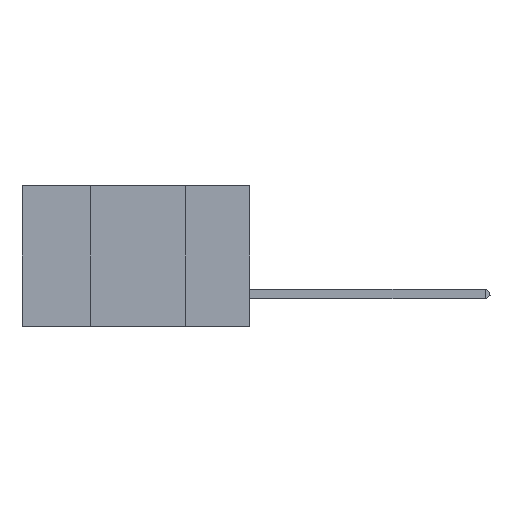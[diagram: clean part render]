
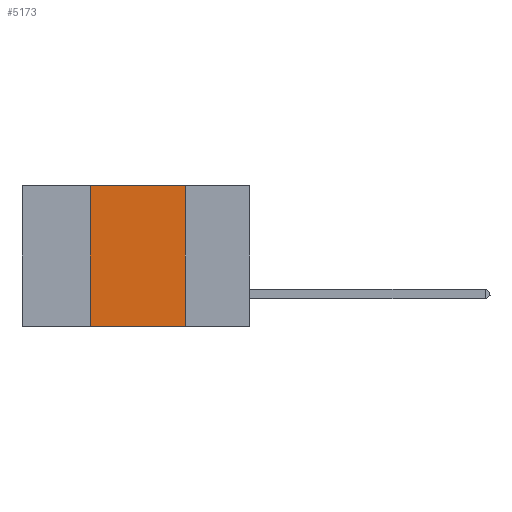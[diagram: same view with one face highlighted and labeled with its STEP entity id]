
A CAD part, left-side view. The second image highlights one B-rep face of the part: STEP entity #5173.
In plain terms, the highlighted planar face has unit normal (-1, 0, 0).
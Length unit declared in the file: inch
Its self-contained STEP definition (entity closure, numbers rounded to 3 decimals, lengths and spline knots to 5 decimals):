
#3717 = CARTESIAN_POINT ( 'NONE',  ( 0., 0.17, -0.37 ) ) ;
#4287 = ORIENTED_EDGE ( 'NONE', *, *, #43970, .F. ) ;
#4582 = PLANE ( 'NONE',  #5928 ) ;
#4859 = CARTESIAN_POINT ( 'NONE',  ( 0., 0.17, 0. ) ) ;
#5173 = ADVANCED_FACE ( 'NONE', ( #27653 ), #4582, .F. ) ;
#5928 = AXIS2_PLACEMENT_3D ( 'NONE', #19264, #23819, #9430 ) ;
#8566 = CARTESIAN_POINT ( 'NONE',  ( 0., 0.17, 0. ) ) ;
#9430 = DIRECTION ( 'NONE',  ( 0., 0., -1. ) ) ;
#11732 = VECTOR ( 'NONE', #38789, 39.37008 ) ;
#11736 = VECTOR ( 'NONE', #12236, 39.37008 ) ;
#12236 = DIRECTION ( 'NONE',  ( 0., -1., 0. ) ) ;
#12929 = VERTEX_POINT ( 'NONE', #45999 ) ;
#15854 = CARTESIAN_POINT ( 'NONE',  ( 0., 0.6, -0.37 ) ) ;
#19030 = VERTEX_POINT ( 'NONE', #3717 ) ;
#19264 = CARTESIAN_POINT ( 'NONE',  ( 0., 0.6, 0. ) ) ;
#20311 = EDGE_CURVE ( 'NONE', #21935, #45331, #34620, .T. ) ;
#21935 = VERTEX_POINT ( 'NONE', #44883 ) ;
#22115 = EDGE_CURVE ( 'NONE', #45331, #19030, #37363, .T. ) ;
#22333 = ORIENTED_EDGE ( 'NONE', *, *, #20311, .F. ) ;
#22839 = LINE ( 'NONE', #15854, #11736 ) ;
#23819 = DIRECTION ( 'NONE',  ( 1., 0., 0. ) ) ;
#27300 = LINE ( 'NONE', #35301, #29658 ) ;
#27653 = FACE_OUTER_BOUND ( 'NONE', #36079, .T. ) ;
#29658 = VECTOR ( 'NONE', #39220, 39.37008 ) ;
#34044 = VECTOR ( 'NONE', #42237, 39.37008 ) ;
#34620 = LINE ( 'NONE', #34877, #34044 ) ;
#34877 = CARTESIAN_POINT ( 'NONE',  ( 0., 0.6, 0. ) ) ;
#35301 = CARTESIAN_POINT ( 'NONE',  ( 0., 0.42, 0. ) ) ;
#36079 = EDGE_LOOP ( 'NONE', ( #37472, #22333, #4287, #46517 ) ) ;
#36971 = EDGE_CURVE ( 'NONE', #12929, #19030, #22839, .T. ) ;
#37363 = LINE ( 'NONE', #8566, #11732 ) ;
#37472 = ORIENTED_EDGE ( 'NONE', *, *, #22115, .F. ) ;
#38789 = DIRECTION ( 'NONE',  ( 0., 0., -1. ) ) ;
#39220 = DIRECTION ( 'NONE',  ( 0., 0., 1. ) ) ;
#42237 = DIRECTION ( 'NONE',  ( 0., -1., 0. ) ) ;
#43970 = EDGE_CURVE ( 'NONE', #12929, #21935, #27300, .T. ) ;
#44883 = CARTESIAN_POINT ( 'NONE',  ( 0., 0.42, 0. ) ) ;
#45331 = VERTEX_POINT ( 'NONE', #4859 ) ;
#45999 = CARTESIAN_POINT ( 'NONE',  ( 0., 0.42, -0.37 ) ) ;
#46517 = ORIENTED_EDGE ( 'NONE', *, *, #36971, .T. ) ;
